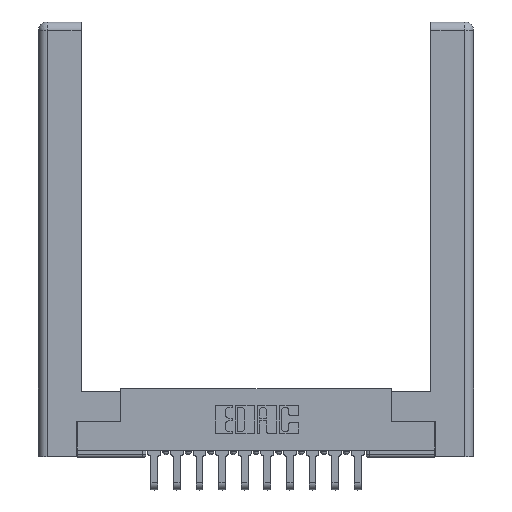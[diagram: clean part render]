
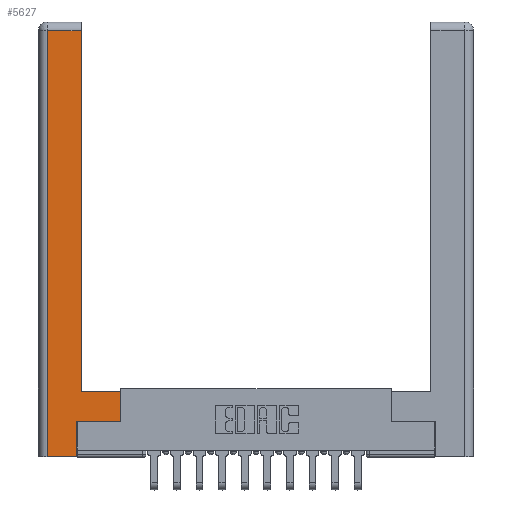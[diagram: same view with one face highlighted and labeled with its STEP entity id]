
A CAD part, top view. The second image highlights one B-rep face of the part: STEP entity #5627.
In plain terms, the highlighted planar face has unit normal (0, 0, 1).
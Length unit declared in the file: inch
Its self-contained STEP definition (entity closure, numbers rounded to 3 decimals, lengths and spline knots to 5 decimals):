
#95 = CARTESIAN_POINT ( 'NONE',  ( 0.0615, 0., 0. ) ) ;
#253 = VERTEX_POINT ( 'NONE', #8868 ) ;
#490 = ORIENTED_EDGE ( 'NONE', *, *, #11619, .T. ) ;
#624 = EDGE_CURVE ( 'NONE', #4102, #2810, #14567, .T. ) ;
#1088 = ORIENTED_EDGE ( 'NONE', *, *, #11659, .T. ) ;
#1138 = CARTESIAN_POINT ( 'NONE',  ( 0.0615, 0., 0. ) ) ;
#1237 = AXIS2_PLACEMENT_3D ( 'NONE', #9895, #6133, #16681 ) ;
#1296 = VERTEX_POINT ( 'NONE', #6241 ) ;
#1469 = CARTESIAN_POINT ( 'NONE',  ( 0.295, 0.45, 0. ) ) ;
#1909 = VECTOR ( 'NONE', #14046, 39.37008 ) ;
#2117 = LINE ( 'NONE', #14128, #6306 ) ;
#2461 = CARTESIAN_POINT ( 'NONE',  ( 0.265, 0.245, 0. ) ) ;
#2810 = VERTEX_POINT ( 'NONE', #3912 ) ;
#2890 = LINE ( 'NONE', #15930, #4884 ) ;
#3598 = DIRECTION ( 'NONE',  ( -1., 0., 0. ) ) ;
#3864 = LINE ( 'NONE', #1138, #8471 ) ;
#3869 = VECTOR ( 'NONE', #3598, 39.37008 ) ;
#3912 = CARTESIAN_POINT ( 'NONE',  ( 0.265, 0., 0. ) ) ;
#4061 = VECTOR ( 'NONE', #16887, 39.37008 ) ;
#4102 = VERTEX_POINT ( 'NONE', #95 ) ;
#4248 = DIRECTION ( 'NONE',  ( 1., 0., 0. ) ) ;
#4758 = CARTESIAN_POINT ( 'NONE',  ( 0.265, 0.245, 0. ) ) ;
#4836 = PLANE ( 'NONE',  #1237 ) ;
#4884 = VECTOR ( 'NONE', #10683, 39.37008 ) ;
#5627 = ADVANCED_FACE ( 'NONE', ( #12535 ), #4836, .F. ) ;
#6133 = DIRECTION ( 'NONE',  ( 0., 0., -1. ) ) ;
#6241 = CARTESIAN_POINT ( 'NONE',  ( 0.565, 0.245, 0. ) ) ;
#6263 = LINE ( 'NONE', #8923, #3869 ) ;
#6306 = VECTOR ( 'NONE', #15416, 39.37008 ) ;
#6757 = LINE ( 'NONE', #11959, #4061 ) ;
#7490 = CARTESIAN_POINT ( 'NONE',  ( 0.565, 0.45, 0. ) ) ;
#7927 = ORIENTED_EDGE ( 'NONE', *, *, #14293, .T. ) ;
#8331 = VERTEX_POINT ( 'NONE', #11018 ) ;
#8471 = VECTOR ( 'NONE', #9409, 39.37008 ) ;
#8656 = VERTEX_POINT ( 'NONE', #7490 ) ;
#8868 = CARTESIAN_POINT ( 'NONE',  ( 0.295, 2.94, 0. ) ) ;
#8923 = CARTESIAN_POINT ( 'NONE',  ( 0.0615, 2.94, 0. ) ) ;
#9409 = DIRECTION ( 'NONE',  ( 0., -1., 0. ) ) ;
#9592 = ORIENTED_EDGE ( 'NONE', *, *, #624, .T. ) ;
#9789 = ORIENTED_EDGE ( 'NONE', *, *, #13339, .T. ) ;
#9895 = CARTESIAN_POINT ( 'NONE',  ( 0., 0., 0. ) ) ;
#9957 = VECTOR ( 'NONE', #10166, 39.37008 ) ;
#10110 = EDGE_CURVE ( 'NONE', #1296, #8656, #6757, .T. ) ;
#10158 = EDGE_CURVE ( 'NONE', #15733, #1296, #2890, .T. ) ;
#10166 = DIRECTION ( 'NONE',  ( 0., 1., 0. ) ) ;
#10683 = DIRECTION ( 'NONE',  ( 1., 0., 0. ) ) ;
#10955 = ORIENTED_EDGE ( 'NONE', *, *, #10158, .T. ) ;
#11018 = CARTESIAN_POINT ( 'NONE',  ( 0.0615, 2.94, 0. ) ) ;
#11261 = VECTOR ( 'NONE', #4248, 39.37008 ) ;
#11374 = EDGE_CURVE ( 'NONE', #8331, #4102, #3864, .T. ) ;
#11428 = LINE ( 'NONE', #4758, #9957 ) ;
#11619 = EDGE_CURVE ( 'NONE', #16736, #253, #13768, .T. ) ;
#11659 = EDGE_CURVE ( 'NONE', #8656, #16736, #2117, .T. ) ;
#11959 = CARTESIAN_POINT ( 'NONE',  ( 0.565, 0.45, 0. ) ) ;
#12535 = FACE_OUTER_BOUND ( 'NONE', #12922, .T. ) ;
#12922 = EDGE_LOOP ( 'NONE', ( #490, #9789, #13880, #9592, #7927, #10955, #16914, #1088 ) ) ;
#13339 = EDGE_CURVE ( 'NONE', #253, #8331, #6263, .T. ) ;
#13768 = LINE ( 'NONE', #15324, #1909 ) ;
#13880 = ORIENTED_EDGE ( 'NONE', *, *, #11374, .T. ) ;
#14046 = DIRECTION ( 'NONE',  ( 0., 1., 0. ) ) ;
#14128 = CARTESIAN_POINT ( 'NONE',  ( 0.295, 0.45, 0. ) ) ;
#14293 = EDGE_CURVE ( 'NONE', #2810, #15733, #11428, .T. ) ;
#14567 = LINE ( 'NONE', #16011, #11261 ) ;
#15324 = CARTESIAN_POINT ( 'NONE',  ( 0.295, 3., 0. ) ) ;
#15416 = DIRECTION ( 'NONE',  ( -1., 0., 0. ) ) ;
#15733 = VERTEX_POINT ( 'NONE', #2461 ) ;
#15930 = CARTESIAN_POINT ( 'NONE',  ( 0.565, 0.245, 0. ) ) ;
#16011 = CARTESIAN_POINT ( 'NONE',  ( 0.265, 0., 0. ) ) ;
#16681 = DIRECTION ( 'NONE',  ( -1., 0., 0. ) ) ;
#16736 = VERTEX_POINT ( 'NONE', #1469 ) ;
#16887 = DIRECTION ( 'NONE',  ( 0., 1., 0. ) ) ;
#16914 = ORIENTED_EDGE ( 'NONE', *, *, #10110, .T. ) ;
